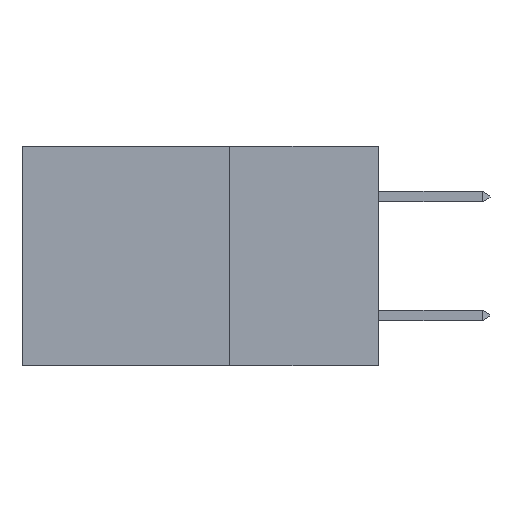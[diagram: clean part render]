
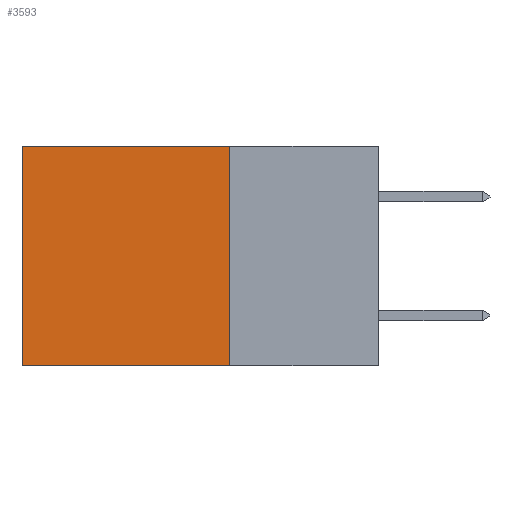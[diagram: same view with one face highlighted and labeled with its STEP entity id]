
A CAD part, left-side view. The second image highlights one B-rep face of the part: STEP entity #3593.
In plain terms, the highlighted planar face has unit normal (-1, 0, 0).
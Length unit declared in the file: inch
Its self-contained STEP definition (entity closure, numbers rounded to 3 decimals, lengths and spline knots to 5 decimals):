
#66 = DIRECTION ( 'NONE',  ( 1., 0., 0. ) ) ;
#429 = EDGE_CURVE ( 'NONE', #4998, #19385, #17811, .T. ) ;
#2099 = EDGE_CURVE ( 'NONE', #4998, #19059, #4533, .T. ) ;
#2585 = LINE ( 'NONE', #21020, #11224 ) ;
#3593 = ADVANCED_FACE ( 'NONE', ( #23591 ), #15477, .F. ) ;
#4171 = VERTEX_POINT ( 'NONE', #22561 ) ;
#4522 = VECTOR ( 'NONE', #14795, 39.37008 ) ;
#4533 = LINE ( 'NONE', #4566, #15753 ) ;
#4566 = CARTESIAN_POINT ( 'NONE',  ( 0.298, 0.25, 0. ) ) ;
#4807 = CARTESIAN_POINT ( 'NONE',  ( 0.298, 0.6, 0. ) ) ;
#4998 = VERTEX_POINT ( 'NONE', #6474 ) ;
#6474 = CARTESIAN_POINT ( 'NONE',  ( 0.298, 0.25, 0. ) ) ;
#7217 = VECTOR ( 'NONE', #18216, 39.37008 ) ;
#8438 = CARTESIAN_POINT ( 'NONE',  ( 0.298, 0.25, -0.37 ) ) ;
#10412 = CARTESIAN_POINT ( 'NONE',  ( 0.298, 0.25, 0. ) ) ;
#10782 = LINE ( 'NONE', #8438, #4522 ) ;
#10959 = ORIENTED_EDGE ( 'NONE', *, *, #24077, .F. ) ;
#11224 = VECTOR ( 'NONE', #18985, 39.37008 ) ;
#14011 = ORIENTED_EDGE ( 'NONE', *, *, #18176, .T. ) ;
#14185 = DIRECTION ( 'NONE',  ( 0., 1., 0. ) ) ;
#14795 = DIRECTION ( 'NONE',  ( 0., 1., 0. ) ) ;
#15010 = ORIENTED_EDGE ( 'NONE', *, *, #429, .F. ) ;
#15477 = PLANE ( 'NONE',  #17873 ) ;
#15753 = VECTOR ( 'NONE', #14185, 39.37008 ) ;
#17811 = LINE ( 'NONE', #18249, #7217 ) ;
#17873 = AXIS2_PLACEMENT_3D ( 'NONE', #10412, #66, #18246 ) ;
#18176 = EDGE_CURVE ( 'NONE', #19059, #4171, #2585, .T. ) ;
#18216 = DIRECTION ( 'NONE',  ( 0., 0., -1. ) ) ;
#18246 = DIRECTION ( 'NONE',  ( 0., 0., -1. ) ) ;
#18249 = CARTESIAN_POINT ( 'NONE',  ( 0.298, 0.25, 0. ) ) ;
#18985 = DIRECTION ( 'NONE',  ( 0., 0., -1. ) ) ;
#19059 = VERTEX_POINT ( 'NONE', #4807 ) ;
#19385 = VERTEX_POINT ( 'NONE', #20566 ) ;
#19758 = EDGE_LOOP ( 'NONE', ( #14011, #10959, #15010, #20113 ) ) ;
#20113 = ORIENTED_EDGE ( 'NONE', *, *, #2099, .T. ) ;
#20566 = CARTESIAN_POINT ( 'NONE',  ( 0.298, 0.25, -0.37 ) ) ;
#21020 = CARTESIAN_POINT ( 'NONE',  ( 0.298, 0.6, 0. ) ) ;
#22561 = CARTESIAN_POINT ( 'NONE',  ( 0.298, 0.6, -0.37 ) ) ;
#23591 = FACE_OUTER_BOUND ( 'NONE', #19758, .T. ) ;
#24077 = EDGE_CURVE ( 'NONE', #19385, #4171, #10782, .T. ) ;
